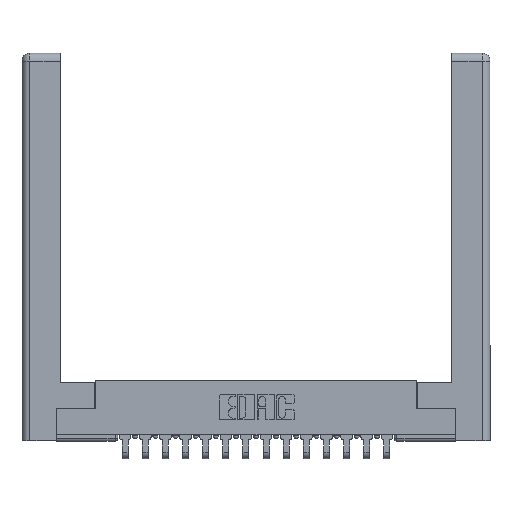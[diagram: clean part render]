
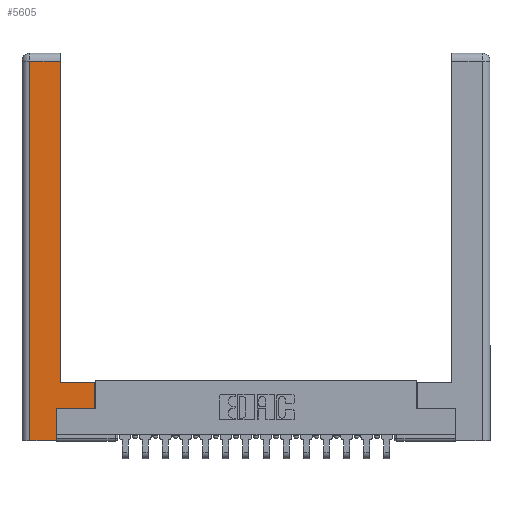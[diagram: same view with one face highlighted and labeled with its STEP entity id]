
A CAD part, top view. The second image highlights one B-rep face of the part: STEP entity #5605.
In plain terms, the highlighted planar face has unit normal (0, 0, 1).
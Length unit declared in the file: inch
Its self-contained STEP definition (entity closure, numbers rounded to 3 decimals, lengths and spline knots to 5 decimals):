
#181 = CARTESIAN_POINT ( 'NONE',  ( 0.565, 0.45, 0. ) ) ;
#416 = CARTESIAN_POINT ( 'NONE',  ( 0.295, 2.94, 0. ) ) ;
#940 = VECTOR ( 'NONE', #16466, 39.37008 ) ;
#1100 = ORIENTED_EDGE ( 'NONE', *, *, #17602, .T. ) ;
#1639 = VERTEX_POINT ( 'NONE', #8415 ) ;
#1727 = CARTESIAN_POINT ( 'NONE',  ( 0.0615, 2.94, 0. ) ) ;
#1750 = VECTOR ( 'NONE', #6917, 39.37008 ) ;
#2244 = FACE_OUTER_BOUND ( 'NONE', #12408, .T. ) ;
#2545 = EDGE_CURVE ( 'NONE', #1639, #4806, #10707, .T. ) ;
#2602 = ORIENTED_EDGE ( 'NONE', *, *, #10923, .T. ) ;
#2780 = DIRECTION ( 'NONE',  ( 0., 0., -1. ) ) ;
#4409 = VERTEX_POINT ( 'NONE', #13926 ) ;
#4476 = CARTESIAN_POINT ( 'NONE',  ( 0.265, 0., 0. ) ) ;
#4574 = DIRECTION ( 'NONE',  ( -1., 0., 0. ) ) ;
#4806 = VERTEX_POINT ( 'NONE', #10632 ) ;
#5282 = EDGE_CURVE ( 'NONE', #16670, #16229, #16302, .T. ) ;
#5373 = LINE ( 'NONE', #10922, #12369 ) ;
#5605 = ADVANCED_FACE ( 'NONE', ( #2244 ), #14234, .F. ) ;
#5949 = VECTOR ( 'NONE', #13178, 39.37008 ) ;
#6338 = VERTEX_POINT ( 'NONE', #416 ) ;
#6414 = CARTESIAN_POINT ( 'NONE',  ( 0.0615, 0., 0. ) ) ;
#6542 = DIRECTION ( 'NONE',  ( 0., -1., 0. ) ) ;
#6917 = DIRECTION ( 'NONE',  ( 1., 0., 0. ) ) ;
#7192 = VECTOR ( 'NONE', #15699, 39.37008 ) ;
#7336 = ORIENTED_EDGE ( 'NONE', *, *, #2545, .T. ) ;
#7376 = CARTESIAN_POINT ( 'NONE',  ( 0.295, 0.45, 0. ) ) ;
#7508 = LINE ( 'NONE', #6414, #11673 ) ;
#7937 = VECTOR ( 'NONE', #4574, 39.37008 ) ;
#8117 = AXIS2_PLACEMENT_3D ( 'NONE', #16878, #2780, #8495 ) ;
#8348 = VERTEX_POINT ( 'NONE', #12070 ) ;
#8415 = CARTESIAN_POINT ( 'NONE',  ( 0.565, 0.245, 0. ) ) ;
#8495 = DIRECTION ( 'NONE',  ( -1., 0., 0. ) ) ;
#8608 = ORIENTED_EDGE ( 'NONE', *, *, #5282, .T. ) ;
#8679 = VECTOR ( 'NONE', #10584, 39.37008 ) ;
#9720 = EDGE_CURVE ( 'NONE', #8348, #6338, #5373, .T. ) ;
#10206 = LINE ( 'NONE', #13334, #8679 ) ;
#10578 = ORIENTED_EDGE ( 'NONE', *, *, #9720, .T. ) ;
#10584 = DIRECTION ( 'NONE',  ( 1., 0., 0. ) ) ;
#10632 = CARTESIAN_POINT ( 'NONE',  ( 0.565, 0.45, 0. ) ) ;
#10707 = LINE ( 'NONE', #181, #7192 ) ;
#10922 = CARTESIAN_POINT ( 'NONE',  ( 0.295, 3., 0. ) ) ;
#10923 = EDGE_CURVE ( 'NONE', #13107, #4409, #7508, .T. ) ;
#11343 = EDGE_CURVE ( 'NONE', #4806, #8348, #13185, .T. ) ;
#11673 = VECTOR ( 'NONE', #6542, 39.37008 ) ;
#11890 = CARTESIAN_POINT ( 'NONE',  ( 0.0615, 2.94, 0. ) ) ;
#12070 = CARTESIAN_POINT ( 'NONE',  ( 0.295, 0.45, 0. ) ) ;
#12369 = VECTOR ( 'NONE', #15245, 39.37008 ) ;
#12405 = ORIENTED_EDGE ( 'NONE', *, *, #11343, .T. ) ;
#12408 = EDGE_LOOP ( 'NONE', ( #10578, #1100, #2602, #14247, #8608, #17989, #7336, #12405 ) ) ;
#13107 = VERTEX_POINT ( 'NONE', #1727 ) ;
#13178 = DIRECTION ( 'NONE',  ( -1., 0., 0. ) ) ;
#13185 = LINE ( 'NONE', #7376, #7937 ) ;
#13334 = CARTESIAN_POINT ( 'NONE',  ( 0.565, 0.245, 0. ) ) ;
#13926 = CARTESIAN_POINT ( 'NONE',  ( 0.0615, 0., 0. ) ) ;
#14234 = PLANE ( 'NONE',  #8117 ) ;
#14247 = ORIENTED_EDGE ( 'NONE', *, *, #17914, .T. ) ;
#14458 = CARTESIAN_POINT ( 'NONE',  ( 0.265, 0.245, 0. ) ) ;
#15245 = DIRECTION ( 'NONE',  ( 0., 1., 0. ) ) ;
#15298 = CARTESIAN_POINT ( 'NONE',  ( 0.265, 0., 0. ) ) ;
#15300 = EDGE_CURVE ( 'NONE', #16229, #1639, #10206, .T. ) ;
#15699 = DIRECTION ( 'NONE',  ( 0., 1., 0. ) ) ;
#16229 = VERTEX_POINT ( 'NONE', #14458 ) ;
#16302 = LINE ( 'NONE', #16345, #940 ) ;
#16324 = LINE ( 'NONE', #15298, #1750 ) ;
#16345 = CARTESIAN_POINT ( 'NONE',  ( 0.265, 0.245, 0. ) ) ;
#16466 = DIRECTION ( 'NONE',  ( 0., 1., 0. ) ) ;
#16670 = VERTEX_POINT ( 'NONE', #4476 ) ;
#16878 = CARTESIAN_POINT ( 'NONE',  ( 0., 0., 0. ) ) ;
#17131 = LINE ( 'NONE', #11890, #5949 ) ;
#17602 = EDGE_CURVE ( 'NONE', #6338, #13107, #17131, .T. ) ;
#17914 = EDGE_CURVE ( 'NONE', #4409, #16670, #16324, .T. ) ;
#17989 = ORIENTED_EDGE ( 'NONE', *, *, #15300, .T. ) ;
